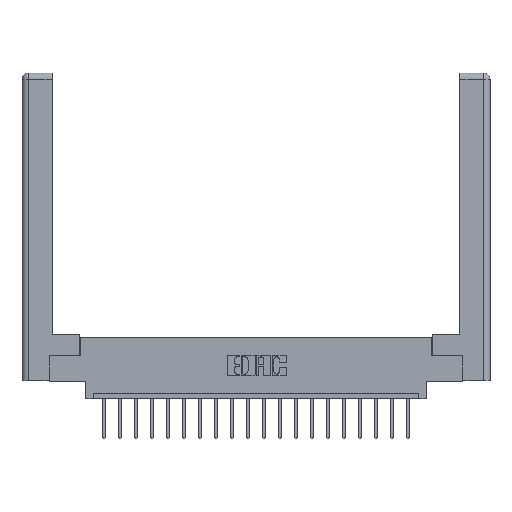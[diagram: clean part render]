
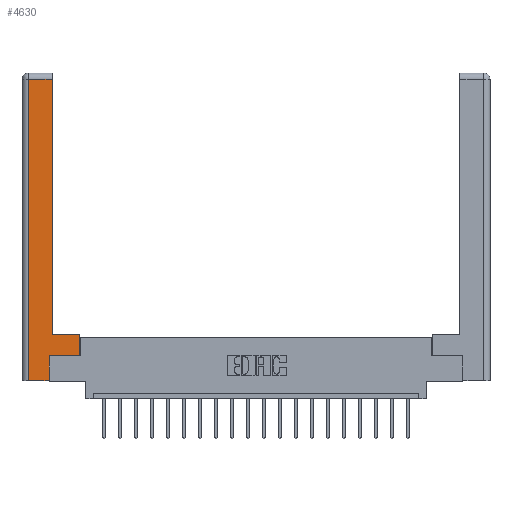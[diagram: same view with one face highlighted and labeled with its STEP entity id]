
A CAD part, top view. The second image highlights one B-rep face of the part: STEP entity #4630.
In plain terms, the highlighted planar face has unit normal (0, 0, 1).
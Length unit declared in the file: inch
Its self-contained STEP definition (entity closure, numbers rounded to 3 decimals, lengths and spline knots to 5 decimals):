
#80 = CARTESIAN_POINT ( 'NONE',  ( 0., 0., 0. ) ) ;
#165 = VECTOR ( 'NONE', #16845, 39.37008 ) ;
#1771 = CARTESIAN_POINT ( 'NONE',  ( 0.295, 0.45, 0. ) ) ;
#1895 = CARTESIAN_POINT ( 'NONE',  ( 0.265, 0., 0. ) ) ;
#1914 = CARTESIAN_POINT ( 'NONE',  ( 0.295, 3., 0. ) ) ;
#2510 = EDGE_CURVE ( 'NONE', #4114, #4745, #6667, .T. ) ;
#2596 = CARTESIAN_POINT ( 'NONE',  ( 0.265, 0.245, 0. ) ) ;
#2805 = CARTESIAN_POINT ( 'NONE',  ( 0.265, 0., 0. ) ) ;
#2966 = EDGE_CURVE ( 'NONE', #13463, #20505, #13474, .T. ) ;
#3009 = EDGE_CURVE ( 'NONE', #20505, #17624, #20424, .T. ) ;
#3498 = CARTESIAN_POINT ( 'NONE',  ( 0.565, 0.245, 0. ) ) ;
#3948 = LINE ( 'NONE', #8419, #8833 ) ;
#4058 = DIRECTION ( 'NONE',  ( -1., 0., 0. ) ) ;
#4075 = CARTESIAN_POINT ( 'NONE',  ( 0.0615, 0., 0. ) ) ;
#4114 = VERTEX_POINT ( 'NONE', #11004 ) ;
#4630 = ADVANCED_FACE ( 'NONE', ( #16893 ), #14252, .F. ) ;
#4710 = CARTESIAN_POINT ( 'NONE',  ( 0.0615, 0., 0. ) ) ;
#4745 = VERTEX_POINT ( 'NONE', #6328 ) ;
#5094 = ORIENTED_EDGE ( 'NONE', *, *, #18455, .T. ) ;
#5598 = EDGE_CURVE ( 'NONE', #13241, #13463, #13065, .T. ) ;
#5978 = VECTOR ( 'NONE', #19941, 39.37008 ) ;
#6328 = CARTESIAN_POINT ( 'NONE',  ( 0.295, 0.45, 0. ) ) ;
#6394 = ORIENTED_EDGE ( 'NONE', *, *, #5598, .T. ) ;
#6454 = DIRECTION ( 'NONE',  ( -1., 0., 0. ) ) ;
#6589 = DIRECTION ( 'NONE',  ( 0., 1., 0. ) ) ;
#6667 = LINE ( 'NONE', #1771, #18769 ) ;
#6681 = VECTOR ( 'NONE', #4058, 39.37008 ) ;
#6881 = LINE ( 'NONE', #18424, #165 ) ;
#7157 = CARTESIAN_POINT ( 'NONE',  ( 0.0615, 2.94, 0. ) ) ;
#7832 = DIRECTION ( 'NONE',  ( 0., 0., -1. ) ) ;
#7907 = DIRECTION ( 'NONE',  ( -1., 0., 0. ) ) ;
#8419 = CARTESIAN_POINT ( 'NONE',  ( 0.565, 0.45, 0. ) ) ;
#8456 = VECTOR ( 'NONE', #6589, 39.37008 ) ;
#8728 = CARTESIAN_POINT ( 'NONE',  ( 0.0615, 2.94, 0. ) ) ;
#8778 = EDGE_CURVE ( 'NONE', #4745, #13241, #9444, .T. ) ;
#8833 = VECTOR ( 'NONE', #17977, 39.37008 ) ;
#9011 = VECTOR ( 'NONE', #9307, 39.37008 ) ;
#9307 = DIRECTION ( 'NONE',  ( 0., -1., 0. ) ) ;
#9444 = LINE ( 'NONE', #1914, #8456 ) ;
#10062 = EDGE_LOOP ( 'NONE', ( #10570, #6394, #19273, #13044, #11175, #15260, #5094, #15152 ) ) ;
#10570 = ORIENTED_EDGE ( 'NONE', *, *, #8778, .T. ) ;
#11004 = CARTESIAN_POINT ( 'NONE',  ( 0.565, 0.45, 0. ) ) ;
#11175 = ORIENTED_EDGE ( 'NONE', *, *, #12506, .T. ) ;
#11376 = DIRECTION ( 'NONE',  ( 1., 0., 0. ) ) ;
#12026 = CARTESIAN_POINT ( 'NONE',  ( 0.265, 0.245, 0. ) ) ;
#12506 = EDGE_CURVE ( 'NONE', #17624, #15968, #18592, .T. ) ;
#13044 = ORIENTED_EDGE ( 'NONE', *, *, #3009, .T. ) ;
#13065 = LINE ( 'NONE', #7157, #6681 ) ;
#13241 = VERTEX_POINT ( 'NONE', #16104 ) ;
#13344 = AXIS2_PLACEMENT_3D ( 'NONE', #80, #7832, #7907 ) ;
#13463 = VERTEX_POINT ( 'NONE', #8728 ) ;
#13474 = LINE ( 'NONE', #4710, #9011 ) ;
#14252 = PLANE ( 'NONE',  #13344 ) ;
#14581 = EDGE_CURVE ( 'NONE', #15968, #18653, #6881, .T. ) ;
#15152 = ORIENTED_EDGE ( 'NONE', *, *, #2510, .T. ) ;
#15260 = ORIENTED_EDGE ( 'NONE', *, *, #14581, .T. ) ;
#15968 = VERTEX_POINT ( 'NONE', #2596 ) ;
#16104 = CARTESIAN_POINT ( 'NONE',  ( 0.295, 2.94, 0. ) ) ;
#16845 = DIRECTION ( 'NONE',  ( 1., 0., 0. ) ) ;
#16893 = FACE_OUTER_BOUND ( 'NONE', #10062, .T. ) ;
#17624 = VERTEX_POINT ( 'NONE', #2805 ) ;
#17977 = DIRECTION ( 'NONE',  ( 0., 1., 0. ) ) ;
#18424 = CARTESIAN_POINT ( 'NONE',  ( 0.565, 0.245, 0. ) ) ;
#18455 = EDGE_CURVE ( 'NONE', #18653, #4114, #3948, .T. ) ;
#18592 = LINE ( 'NONE', #12026, #5978 ) ;
#18653 = VERTEX_POINT ( 'NONE', #3498 ) ;
#18769 = VECTOR ( 'NONE', #6454, 39.37008 ) ;
#19273 = ORIENTED_EDGE ( 'NONE', *, *, #2966, .T. ) ;
#19441 = VECTOR ( 'NONE', #11376, 39.37008 ) ;
#19941 = DIRECTION ( 'NONE',  ( 0., 1., 0. ) ) ;
#20424 = LINE ( 'NONE', #1895, #19441 ) ;
#20505 = VERTEX_POINT ( 'NONE', #4075 ) ;
